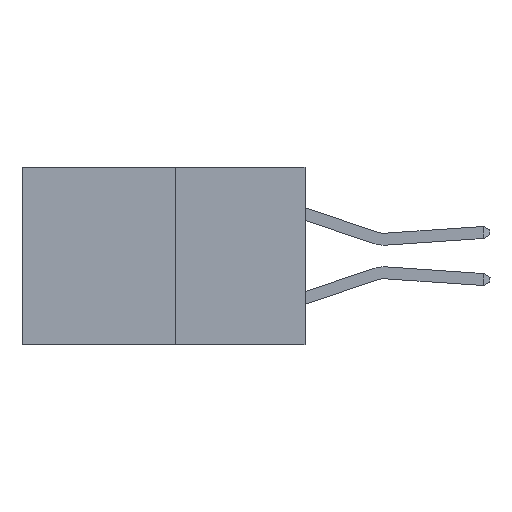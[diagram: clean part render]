
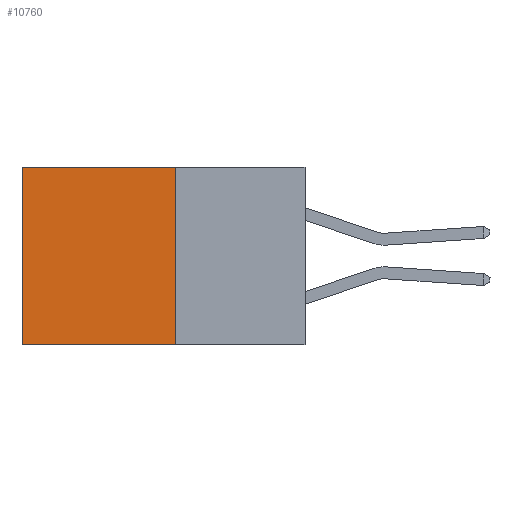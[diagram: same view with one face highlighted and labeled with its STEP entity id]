
A CAD part, left-side view. The second image highlights one B-rep face of the part: STEP entity #10760.
In plain terms, the highlighted planar face has unit normal (-1, 0, 0).
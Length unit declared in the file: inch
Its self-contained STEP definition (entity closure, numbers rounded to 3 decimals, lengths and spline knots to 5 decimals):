
#262 = VERTEX_POINT ( 'NONE', #26098 ) ;
#321 = DIRECTION ( 'NONE',  ( 0., 0., -1. ) ) ;
#1475 = LINE ( 'NONE', #27269, #12284 ) ;
#1566 = VECTOR ( 'NONE', #18788, 39.37008 ) ;
#2507 = VECTOR ( 'NONE', #15233, 39.37008 ) ;
#3667 = CARTESIAN_POINT ( 'NONE',  ( 0.277, 0.27, 0. ) ) ;
#4418 = FACE_OUTER_BOUND ( 'NONE', #19216, .T. ) ;
#6228 = AXIS2_PLACEMENT_3D ( 'NONE', #7182, #22121, #9352 ) ;
#6304 = EDGE_CURVE ( 'NONE', #6671, #8376, #11689, .T. ) ;
#6671 = VERTEX_POINT ( 'NONE', #22786 ) ;
#7182 = CARTESIAN_POINT ( 'NONE',  ( 0.277, 0.27, -0.37 ) ) ;
#7453 = EDGE_CURVE ( 'NONE', #6671, #23683, #8666, .T. ) ;
#8247 = LINE ( 'NONE', #13105, #2507 ) ;
#8376 = VERTEX_POINT ( 'NONE', #14770 ) ;
#8553 = EDGE_CURVE ( 'NONE', #8376, #262, #8247, .T. ) ;
#8666 = LINE ( 'NONE', #3667, #1566 ) ;
#9352 = DIRECTION ( 'NONE',  ( 0., 0., -1. ) ) ;
#9662 = ORIENTED_EDGE ( 'NONE', *, *, #18287, .T. ) ;
#10760 = ADVANCED_FACE ( 'NONE', ( #4418 ), #13586, .F. ) ;
#11689 = LINE ( 'NONE', #13269, #18042 ) ;
#12284 = VECTOR ( 'NONE', #25217, 39.37008 ) ;
#13105 = CARTESIAN_POINT ( 'NONE',  ( 0.277, 0.27, -0.37 ) ) ;
#13269 = CARTESIAN_POINT ( 'NONE',  ( 0.277, 0.27, -0.37 ) ) ;
#13586 = PLANE ( 'NONE',  #6228 ) ;
#14770 = CARTESIAN_POINT ( 'NONE',  ( 0.277, 0.27, -0.37 ) ) ;
#15233 = DIRECTION ( 'NONE',  ( 0., 1., 0. ) ) ;
#18042 = VECTOR ( 'NONE', #321, 39.37008 ) ;
#18287 = EDGE_CURVE ( 'NONE', #23683, #262, #1475, .T. ) ;
#18788 = DIRECTION ( 'NONE',  ( 0., 1., 0. ) ) ;
#19216 = EDGE_LOOP ( 'NONE', ( #9662, #20253, #23497, #20785 ) ) ;
#20253 = ORIENTED_EDGE ( 'NONE', *, *, #8553, .F. ) ;
#20785 = ORIENTED_EDGE ( 'NONE', *, *, #7453, .T. ) ;
#20981 = CARTESIAN_POINT ( 'NONE',  ( 0.277, 0.59, 0. ) ) ;
#22121 = DIRECTION ( 'NONE',  ( 1., 0., 0. ) ) ;
#22786 = CARTESIAN_POINT ( 'NONE',  ( 0.277, 0.27, 0. ) ) ;
#23497 = ORIENTED_EDGE ( 'NONE', *, *, #6304, .F. ) ;
#23683 = VERTEX_POINT ( 'NONE', #20981 ) ;
#25217 = DIRECTION ( 'NONE',  ( 0., 0., -1. ) ) ;
#26098 = CARTESIAN_POINT ( 'NONE',  ( 0.277, 0.59, -0.37 ) ) ;
#27269 = CARTESIAN_POINT ( 'NONE',  ( 0.277, 0.59, -0.37 ) ) ;
